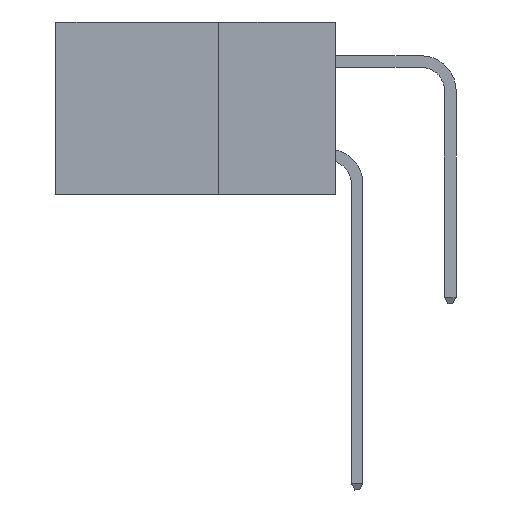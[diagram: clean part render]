
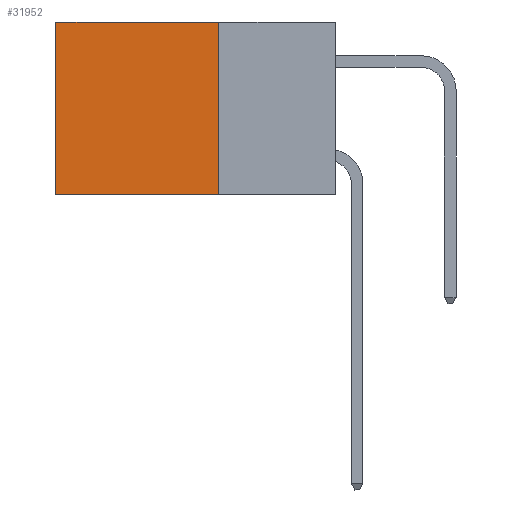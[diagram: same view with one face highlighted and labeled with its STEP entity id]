
A CAD part, left-side view. The second image highlights one B-rep face of the part: STEP entity #31952.
In plain terms, the highlighted planar face has unit normal (-1, 0, 0).
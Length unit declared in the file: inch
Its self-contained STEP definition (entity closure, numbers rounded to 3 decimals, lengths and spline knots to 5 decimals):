
#178 = PLANE ( 'NONE',  #24899 ) ;
#2013 = CARTESIAN_POINT ( 'NONE',  ( 0.2875, 0.6, 0. ) ) ;
#2477 = ORIENTED_EDGE ( 'NONE', *, *, #20734, .T. ) ;
#3190 = CARTESIAN_POINT ( 'NONE',  ( 0.2875, 0.25, 0. ) ) ;
#3652 = DIRECTION ( 'NONE',  ( 0., 1., 0. ) ) ;
#5019 = DIRECTION ( 'NONE',  ( 0., 0., -1. ) ) ;
#5610 = FACE_OUTER_BOUND ( 'NONE', #15254, .T. ) ;
#8237 = VECTOR ( 'NONE', #3652, 39.37008 ) ;
#9311 = CARTESIAN_POINT ( 'NONE',  ( 0.2875, 0.25, 0. ) ) ;
#9838 = ORIENTED_EDGE ( 'NONE', *, *, #35544, .F. ) ;
#10659 = CARTESIAN_POINT ( 'NONE',  ( 0.2875, 0.25, 0. ) ) ;
#12485 = VECTOR ( 'NONE', #16117, 39.37008 ) ;
#14025 = LINE ( 'NONE', #10659, #25608 ) ;
#14034 = VERTEX_POINT ( 'NONE', #2013 ) ;
#14307 = CARTESIAN_POINT ( 'NONE',  ( 0.2875, 0.25, -0.37 ) ) ;
#15254 = EDGE_LOOP ( 'NONE', ( #2477, #37203, #9838, #16175 ) ) ;
#15270 = LINE ( 'NONE', #36917, #12485 ) ;
#15532 = CARTESIAN_POINT ( 'NONE',  ( 0.2875, 0.25, -0.37 ) ) ;
#16117 = DIRECTION ( 'NONE',  ( 0., 0., -1. ) ) ;
#16175 = ORIENTED_EDGE ( 'NONE', *, *, #29174, .T. ) ;
#17328 = EDGE_CURVE ( 'NONE', #31158, #21432, #29458, .T. ) ;
#17893 = DIRECTION ( 'NONE',  ( 1., 0., 0. ) ) ;
#18522 = DIRECTION ( 'NONE',  ( 0., 1., 0. ) ) ;
#20734 = EDGE_CURVE ( 'NONE', #14034, #21432, #15270, .T. ) ;
#21432 = VERTEX_POINT ( 'NONE', #25015 ) ;
#21434 = VERTEX_POINT ( 'NONE', #31641 ) ;
#21612 = VECTOR ( 'NONE', #18522, 39.37008 ) ;
#24899 = AXIS2_PLACEMENT_3D ( 'NONE', #3190, #17893, #29945 ) ;
#25015 = CARTESIAN_POINT ( 'NONE',  ( 0.2875, 0.6, -0.37 ) ) ;
#25608 = VECTOR ( 'NONE', #5019, 39.37008 ) ;
#29174 = EDGE_CURVE ( 'NONE', #21434, #14034, #37051, .T. ) ;
#29458 = LINE ( 'NONE', #15532, #21612 ) ;
#29945 = DIRECTION ( 'NONE',  ( 0., 0., -1. ) ) ;
#31158 = VERTEX_POINT ( 'NONE', #14307 ) ;
#31641 = CARTESIAN_POINT ( 'NONE',  ( 0.2875, 0.25, 0. ) ) ;
#31952 = ADVANCED_FACE ( 'NONE', ( #5610 ), #178, .F. ) ;
#35544 = EDGE_CURVE ( 'NONE', #21434, #31158, #14025, .T. ) ;
#36917 = CARTESIAN_POINT ( 'NONE',  ( 0.2875, 0.6, 0. ) ) ;
#37051 = LINE ( 'NONE', #9311, #8237 ) ;
#37203 = ORIENTED_EDGE ( 'NONE', *, *, #17328, .F. ) ;
